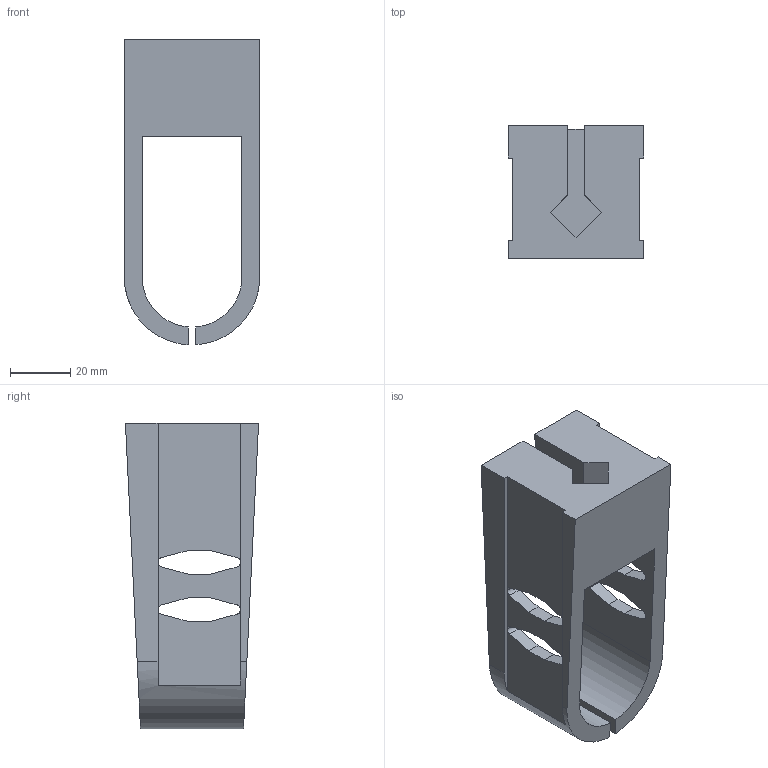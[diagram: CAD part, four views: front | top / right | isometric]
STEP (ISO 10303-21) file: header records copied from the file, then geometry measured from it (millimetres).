
FILE_DESCRIPTION( ( '' ), ' ' );
FILE_NAME( '5dc6e3d09433371275628a6c.step', '2019-11-09T16:05:36', ( '' ), ( '' ), ' ', ' ', ' ' );
FILE_SCHEMA( ( 'AUTOMOTIVE_DESIGN { 1 0 10303 214 1 1 1 1 }' ) );
Length unit declared in the file: metre
Products named in the file (1): Part 1
Bounding box: 44.81 x 44.1 x 101.22 mm (x, y, z)
Volume: 78148 mm3; surface area: 24744.3 mm2
Topology: 1 solids, 1 shells, 73 faces, 225 edges, 150 vertices
Faces by surface type: plane 53, cylinder 20
Entity records: 3119 total; most frequent: ORIENTED_EDGE 450, CARTESIAN_POINT 449, DIRECTION 417, EDGE_CURVE 225, LINE 181, VECTOR 181, VERTEX_POINT 150, AXIS2_PLACEMENT_3D 118
